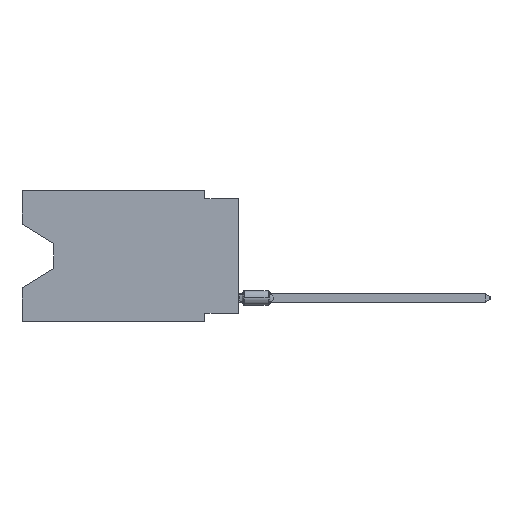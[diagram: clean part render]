
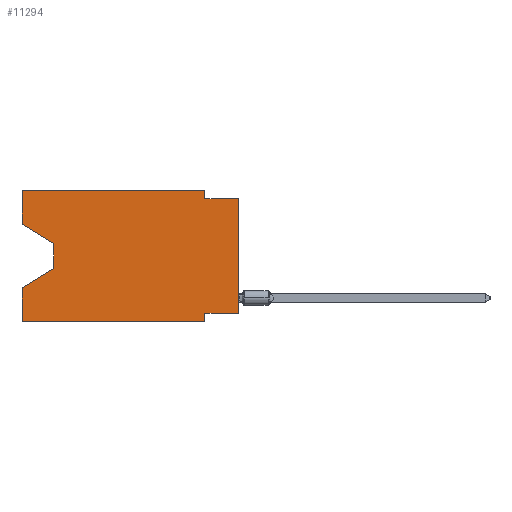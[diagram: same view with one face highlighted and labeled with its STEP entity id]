
A CAD part, left-side view. The second image highlights one B-rep face of the part: STEP entity #11294.
In plain terms, the highlighted planar face has unit normal (-1, 0, 0).
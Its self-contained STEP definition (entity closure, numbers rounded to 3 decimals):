
#21 = EDGE_CURVE ( 'NONE', #40973, #54344, #45229, .T. ) ;
#230 = VECTOR ( 'NONE', #7204, 1000. ) ;
#368 = EDGE_CURVE ( 'NONE', #25027, #23178, #37046, .T. ) ;
#540 = VECTOR ( 'NONE', #31720, 1000. ) ;
#1229 = CARTESIAN_POINT ( 'NONE',  ( 0., 0., -0.635 ) ) ;
#1614 = EDGE_CURVE ( 'NONE', #54344, #31242, #6945, .T. ) ;
#2230 = VECTOR ( 'NONE', #54708, 1000. ) ;
#2427 = CARTESIAN_POINT ( 'NONE',  ( 0., 2.54, 0. ) ) ;
#2779 = VERTEX_POINT ( 'NONE', #23775 ) ;
#3101 = ORIENTED_EDGE ( 'NONE', *, *, #368, .F. ) ;
#4598 = ORIENTED_EDGE ( 'NONE', *, *, #21049, .F. ) ;
#5879 = ORIENTED_EDGE ( 'NONE', *, *, #39516, .F. ) ;
#5880 = CARTESIAN_POINT ( 'NONE',  ( 0., 13.97, -4.013 ) ) ;
#6070 = DIRECTION ( 'NONE',  ( 0., 0., -1. ) ) ;
#6470 = CARTESIAN_POINT ( 'NONE',  ( 0., 16.383, -2.546 ) ) ;
#6471 = CARTESIAN_POINT ( 'NONE',  ( 0., 13.97, -5.893 ) ) ;
#6508 = CARTESIAN_POINT ( 'NONE',  ( 0., 2.54, -9.271 ) ) ;
#6697 = CARTESIAN_POINT ( 'NONE',  ( 0., 2.54, 0. ) ) ;
#6723 = PLANE ( 'NONE',  #9287 ) ;
#6945 = LINE ( 'NONE', #49137, #230 ) ;
#6948 = ORIENTED_EDGE ( 'NONE', *, *, #33260, .F. ) ;
#7204 = DIRECTION ( 'NONE',  ( 0., 0., -1. ) ) ;
#7485 = ORIENTED_EDGE ( 'NONE', *, *, #21, .T. ) ;
#7866 = EDGE_CURVE ( 'NONE', #23178, #40354, #52392, .T. ) ;
#8646 = EDGE_CURVE ( 'NONE', #16126, #40354, #11587, .T. ) ;
#9287 = AXIS2_PLACEMENT_3D ( 'NONE', #53128, #19552, #37161 ) ;
#10213 = CARTESIAN_POINT ( 'NONE',  ( 0., 2.54, -0.635 ) ) ;
#11294 = ADVANCED_FACE ( 'NONE', ( #31876 ), #6723, .F. ) ;
#11587 = LINE ( 'NONE', #50716, #43615 ) ;
#11971 = DIRECTION ( 'NONE',  ( 0., -1., 0. ) ) ;
#13296 = DIRECTION ( 'NONE',  ( 0., -1., 0. ) ) ;
#14741 = EDGE_LOOP ( 'NONE', ( #7485, #26407, #19319, #5879, #29074, #6948, #34845, #36777, #27391, #3101, #52431, #4598 ) ) ;
#16126 = VERTEX_POINT ( 'NONE', #20508 ) ;
#16325 = DIRECTION ( 'NONE',  ( 0., 0., 1. ) ) ;
#16466 = DIRECTION ( 'NONE',  ( 0., 0.855, -0.519 ) ) ;
#16662 = DIRECTION ( 'NONE',  ( 0., 1., 0. ) ) ;
#18260 = VECTOR ( 'NONE', #42258, 1000. ) ;
#18276 = DIRECTION ( 'NONE',  ( 0., -1., 0. ) ) ;
#18411 = EDGE_CURVE ( 'NONE', #31242, #54464, #50010, .T. ) ;
#19319 = ORIENTED_EDGE ( 'NONE', *, *, #18411, .T. ) ;
#19552 = DIRECTION ( 'NONE',  ( 1., 0., 0. ) ) ;
#19656 = CARTESIAN_POINT ( 'NONE',  ( 0., 16.383, -9.906 ) ) ;
#19801 = CARTESIAN_POINT ( 'NONE',  ( 0., 13.97, -5.893 ) ) ;
#20075 = CARTESIAN_POINT ( 'NONE',  ( 0., 16.383, 0. ) ) ;
#20352 = CARTESIAN_POINT ( 'NONE',  ( 0., 0., -0.635 ) ) ;
#20508 = CARTESIAN_POINT ( 'NONE',  ( 0., 0., -9.271 ) ) ;
#21049 = EDGE_CURVE ( 'NONE', #40973, #2779, #36448, .T. ) ;
#21654 = LINE ( 'NONE', #36702, #540 ) ;
#22617 = VECTOR ( 'NONE', #13296, 1000. ) ;
#23178 = VERTEX_POINT ( 'NONE', #10213 ) ;
#23775 = CARTESIAN_POINT ( 'NONE',  ( 0., 16.383, 0. ) ) ;
#25027 = VERTEX_POINT ( 'NONE', #6697 ) ;
#25588 = EDGE_CURVE ( 'NONE', #16126, #44370, #46011, .T. ) ;
#26407 = ORIENTED_EDGE ( 'NONE', *, *, #1614, .T. ) ;
#27391 = ORIENTED_EDGE ( 'NONE', *, *, #7866, .F. ) ;
#29074 = ORIENTED_EDGE ( 'NONE', *, *, #42558, .T. ) ;
#29205 = VECTOR ( 'NONE', #6070, 1000. ) ;
#29365 = EDGE_CURVE ( 'NONE', #2779, #25027, #53900, .T. ) ;
#30440 = VECTOR ( 'NONE', #16466, 1000. ) ;
#31242 = VERTEX_POINT ( 'NONE', #6471 ) ;
#31605 = VECTOR ( 'NONE', #11971, 1000. ) ;
#31720 = DIRECTION ( 'NONE',  ( 0., 0., -1. ) ) ;
#31876 = FACE_OUTER_BOUND ( 'NONE', #14741, .T. ) ;
#32524 = DIRECTION ( 'NONE',  ( 0., 0., 1. ) ) ;
#32812 = CARTESIAN_POINT ( 'NONE',  ( 0., 16.383, 0. ) ) ;
#33260 = EDGE_CURVE ( 'NONE', #44370, #33372, #21654, .T. ) ;
#33372 = VERTEX_POINT ( 'NONE', #48473 ) ;
#34845 = ORIENTED_EDGE ( 'NONE', *, *, #25588, .F. ) ;
#35434 = VERTEX_POINT ( 'NONE', #19656 ) ;
#36448 = LINE ( 'NONE', #32812, #54064 ) ;
#36702 = CARTESIAN_POINT ( 'NONE',  ( 0., 2.54, -9.906 ) ) ;
#36777 = ORIENTED_EDGE ( 'NONE', *, *, #8646, .T. ) ;
#37046 = LINE ( 'NONE', #2427, #29205 ) ;
#37161 = DIRECTION ( 'NONE',  ( 0., 0., -1. ) ) ;
#37793 = CARTESIAN_POINT ( 'NONE',  ( 0., 16.383, 0. ) ) ;
#39516 = EDGE_CURVE ( 'NONE', #35434, #54464, #50683, .T. ) ;
#40354 = VERTEX_POINT ( 'NONE', #20352 ) ;
#40973 = VERTEX_POINT ( 'NONE', #6470 ) ;
#42258 = DIRECTION ( 'NONE',  ( 0., 0., 1. ) ) ;
#42558 = EDGE_CURVE ( 'NONE', #35434, #33372, #47111, .T. ) ;
#43615 = VECTOR ( 'NONE', #16325, 1000. ) ;
#44370 = VERTEX_POINT ( 'NONE', #6508 ) ;
#45229 = LINE ( 'NONE', #55266, #2230 ) ;
#45243 = CARTESIAN_POINT ( 'NONE',  ( 0., 16.383, -7.36 ) ) ;
#45384 = VECTOR ( 'NONE', #18276, 1000. ) ;
#46011 = LINE ( 'NONE', #51793, #51423 ) ;
#46541 = CARTESIAN_POINT ( 'NONE',  ( 0., 16.383, -9.906 ) ) ;
#47111 = LINE ( 'NONE', #46541, #22617 ) ;
#48473 = CARTESIAN_POINT ( 'NONE',  ( 0., 2.54, -9.906 ) ) ;
#49137 = CARTESIAN_POINT ( 'NONE',  ( 0., 13.97, -4.013 ) ) ;
#50010 = LINE ( 'NONE', #19801, #30440 ) ;
#50683 = LINE ( 'NONE', #37793, #18260 ) ;
#50716 = CARTESIAN_POINT ( 'NONE',  ( 0., 0., 0. ) ) ;
#51423 = VECTOR ( 'NONE', #16662, 1000. ) ;
#51793 = CARTESIAN_POINT ( 'NONE',  ( 0., 0., -9.271 ) ) ;
#52392 = LINE ( 'NONE', #1229, #45384 ) ;
#52431 = ORIENTED_EDGE ( 'NONE', *, *, #29365, .F. ) ;
#53128 = CARTESIAN_POINT ( 'NONE',  ( 0., 16.383, 0. ) ) ;
#53900 = LINE ( 'NONE', #20075, #31605 ) ;
#54064 = VECTOR ( 'NONE', #32524, 1000. ) ;
#54344 = VERTEX_POINT ( 'NONE', #5880 ) ;
#54464 = VERTEX_POINT ( 'NONE', #45243 ) ;
#54708 = DIRECTION ( 'NONE',  ( 0., -0.855, -0.519 ) ) ;
#55266 = CARTESIAN_POINT ( 'NONE',  ( 0., 16.383, -2.546 ) ) ;
